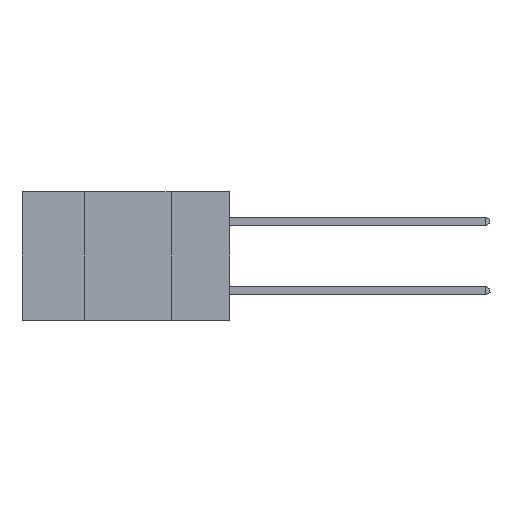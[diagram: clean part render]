
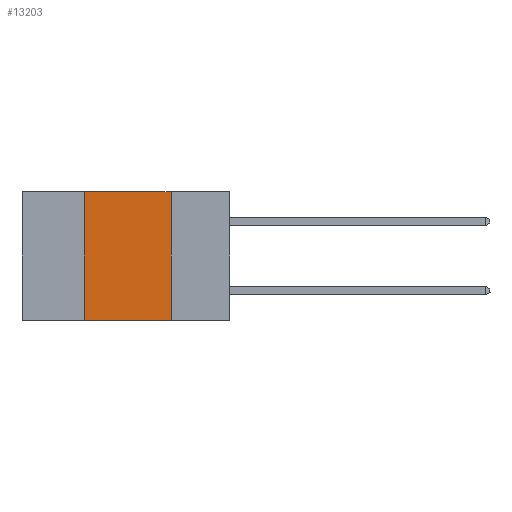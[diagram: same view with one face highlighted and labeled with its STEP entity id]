
A CAD part, left-side view. The second image highlights one B-rep face of the part: STEP entity #13203.
In plain terms, the highlighted planar face has unit normal (-1, 0, 0).
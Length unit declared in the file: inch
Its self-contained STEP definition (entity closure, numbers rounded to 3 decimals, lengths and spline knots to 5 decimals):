
#143 = DIRECTION ( 'NONE',  ( 0., -1., 0. ) ) ;
#871 = EDGE_CURVE ( 'NONE', #14063, #2849, #12852, .T. ) ;
#1173 = DIRECTION ( 'NONE',  ( 0., 0., -1. ) ) ;
#1313 = LINE ( 'NONE', #8298, #11605 ) ;
#1709 = CARTESIAN_POINT ( 'NONE',  ( 0., 0.6, 0. ) ) ;
#1964 = VECTOR ( 'NONE', #6645, 39.37008 ) ;
#1993 = CARTESIAN_POINT ( 'NONE',  ( 0., 0.42, 0. ) ) ;
#2090 = EDGE_CURVE ( 'NONE', #14063, #3198, #7487, .T. ) ;
#2512 = CARTESIAN_POINT ( 'NONE',  ( 0., 0.6, -0.37 ) ) ;
#2826 = VECTOR ( 'NONE', #5160, 39.37008 ) ;
#2849 = VERTEX_POINT ( 'NONE', #14154 ) ;
#3198 = VERTEX_POINT ( 'NONE', #9119 ) ;
#3279 = VERTEX_POINT ( 'NONE', #7682 ) ;
#5160 = DIRECTION ( 'NONE',  ( 0., -1., 0. ) ) ;
#5757 = CARTESIAN_POINT ( 'NONE',  ( 0., 0.42, -0.37 ) ) ;
#5836 = EDGE_LOOP ( 'NONE', ( #12538, #13154, #6142, #6194 ) ) ;
#6142 = ORIENTED_EDGE ( 'NONE', *, *, #871, .F. ) ;
#6194 = ORIENTED_EDGE ( 'NONE', *, *, #2090, .T. ) ;
#6645 = DIRECTION ( 'NONE',  ( 0., 0., 1. ) ) ;
#7487 = LINE ( 'NONE', #2512, #13383 ) ;
#7682 = CARTESIAN_POINT ( 'NONE',  ( 0., 0.17, 0. ) ) ;
#7814 = EDGE_CURVE ( 'NONE', #2849, #3279, #8887, .T. ) ;
#8298 = CARTESIAN_POINT ( 'NONE',  ( 0., 0.17, 0. ) ) ;
#8447 = PLANE ( 'NONE',  #10827 ) ;
#8887 = LINE ( 'NONE', #1709, #2826 ) ;
#9119 = CARTESIAN_POINT ( 'NONE',  ( 0., 0.17, -0.37 ) ) ;
#9625 = CARTESIAN_POINT ( 'NONE',  ( 0., 0.6, 0. ) ) ;
#10827 = AXIS2_PLACEMENT_3D ( 'NONE', #9625, #13192, #14395 ) ;
#11027 = EDGE_CURVE ( 'NONE', #3279, #3198, #1313, .T. ) ;
#11605 = VECTOR ( 'NONE', #1173, 39.37008 ) ;
#12493 = FACE_OUTER_BOUND ( 'NONE', #5836, .T. ) ;
#12538 = ORIENTED_EDGE ( 'NONE', *, *, #11027, .F. ) ;
#12852 = LINE ( 'NONE', #1993, #1964 ) ;
#13154 = ORIENTED_EDGE ( 'NONE', *, *, #7814, .F. ) ;
#13192 = DIRECTION ( 'NONE',  ( 1., 0., 0. ) ) ;
#13203 = ADVANCED_FACE ( 'NONE', ( #12493 ), #8447, .F. ) ;
#13383 = VECTOR ( 'NONE', #143, 39.37008 ) ;
#14063 = VERTEX_POINT ( 'NONE', #5757 ) ;
#14154 = CARTESIAN_POINT ( 'NONE',  ( 0., 0.42, 0. ) ) ;
#14395 = DIRECTION ( 'NONE',  ( 0., 0., -1. ) ) ;
